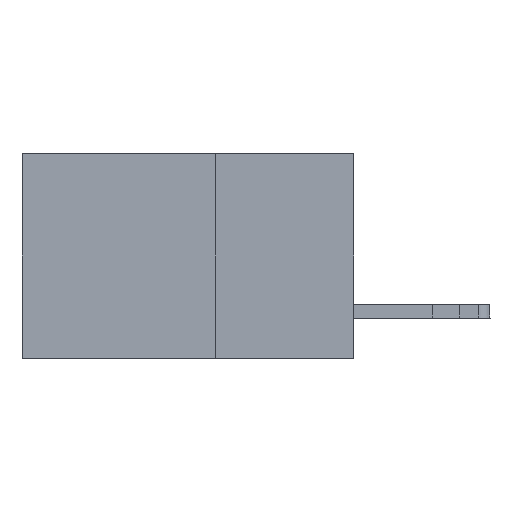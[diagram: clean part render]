
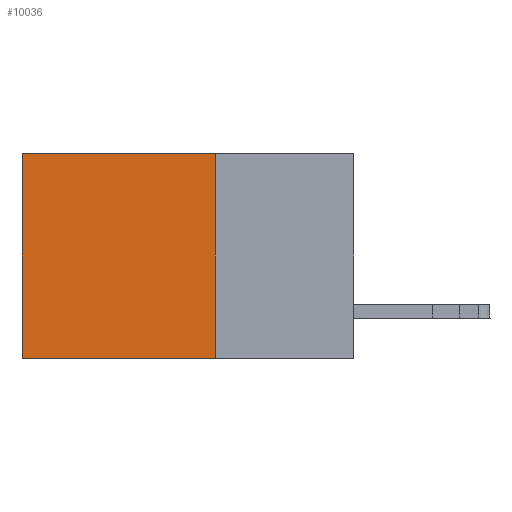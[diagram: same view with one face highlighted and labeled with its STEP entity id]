
A CAD part, left-side view. The second image highlights one B-rep face of the part: STEP entity #10036.
In plain terms, the highlighted planar face has unit normal (-1, 0, 0).
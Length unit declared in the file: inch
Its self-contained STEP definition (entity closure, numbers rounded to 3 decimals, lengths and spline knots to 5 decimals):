
#943 = FACE_OUTER_BOUND ( 'NONE', #2896, .T. ) ;
#953 = AXIS2_PLACEMENT_3D ( 'NONE', #13237, #8783, #16535 ) ;
#2896 = EDGE_LOOP ( 'NONE', ( #18049, #8709, #9176, #18985 ) ) ;
#3865 = VERTEX_POINT ( 'NONE', #19496 ) ;
#3875 = EDGE_CURVE ( 'NONE', #3865, #11580, #5688, .T. ) ;
#4623 = CARTESIAN_POINT ( 'NONE',  ( 0.2875, 0.6, 0. ) ) ;
#4754 = VECTOR ( 'NONE', #14557, 39.37008 ) ;
#5688 = LINE ( 'NONE', #4623, #13193 ) ;
#5706 = CARTESIAN_POINT ( 'NONE',  ( 0.2875, 0.25, -0.37 ) ) ;
#5729 = CARTESIAN_POINT ( 'NONE',  ( 0.2875, 0.25, -0.37 ) ) ;
#5834 = LINE ( 'NONE', #6953, #14433 ) ;
#6208 = DIRECTION ( 'NONE',  ( 0., 0., -1. ) ) ;
#6240 = VECTOR ( 'NONE', #11239, 39.37008 ) ;
#6953 = CARTESIAN_POINT ( 'NONE',  ( 0.2875, 0.25, 0. ) ) ;
#8709 = ORIENTED_EDGE ( 'NONE', *, *, #13001, .F. ) ;
#8783 = DIRECTION ( 'NONE',  ( 1., 0., 0. ) ) ;
#9069 = PLANE ( 'NONE',  #953 ) ;
#9176 = ORIENTED_EDGE ( 'NONE', *, *, #9680, .F. ) ;
#9680 = EDGE_CURVE ( 'NONE', #10641, #10882, #19977, .T. ) ;
#10036 = ADVANCED_FACE ( 'NONE', ( #943 ), #9069, .F. ) ;
#10641 = VERTEX_POINT ( 'NONE', #12647 ) ;
#10882 = VERTEX_POINT ( 'NONE', #5729 ) ;
#11239 = DIRECTION ( 'NONE',  ( 0., 0., -1. ) ) ;
#11580 = VERTEX_POINT ( 'NONE', #17113 ) ;
#11767 = DIRECTION ( 'NONE',  ( 0., 1., 0. ) ) ;
#12647 = CARTESIAN_POINT ( 'NONE',  ( 0.2875, 0.25, 0. ) ) ;
#13001 = EDGE_CURVE ( 'NONE', #10882, #11580, #17701, .T. ) ;
#13193 = VECTOR ( 'NONE', #6208, 39.37008 ) ;
#13237 = CARTESIAN_POINT ( 'NONE',  ( 0.2875, 0.25, 0. ) ) ;
#14433 = VECTOR ( 'NONE', #11767, 39.37008 ) ;
#14557 = DIRECTION ( 'NONE',  ( 0., 1., 0. ) ) ;
#16535 = DIRECTION ( 'NONE',  ( 0., 0., -1. ) ) ;
#17113 = CARTESIAN_POINT ( 'NONE',  ( 0.2875, 0.6, -0.37 ) ) ;
#17701 = LINE ( 'NONE', #5706, #4754 ) ;
#18049 = ORIENTED_EDGE ( 'NONE', *, *, #3875, .T. ) ;
#18985 = ORIENTED_EDGE ( 'NONE', *, *, #21055, .T. ) ;
#19496 = CARTESIAN_POINT ( 'NONE',  ( 0.2875, 0.6, 0. ) ) ;
#19977 = LINE ( 'NONE', #21508, #6240 ) ;
#21055 = EDGE_CURVE ( 'NONE', #10641, #3865, #5834, .T. ) ;
#21508 = CARTESIAN_POINT ( 'NONE',  ( 0.2875, 0.25, 0. ) ) ;
